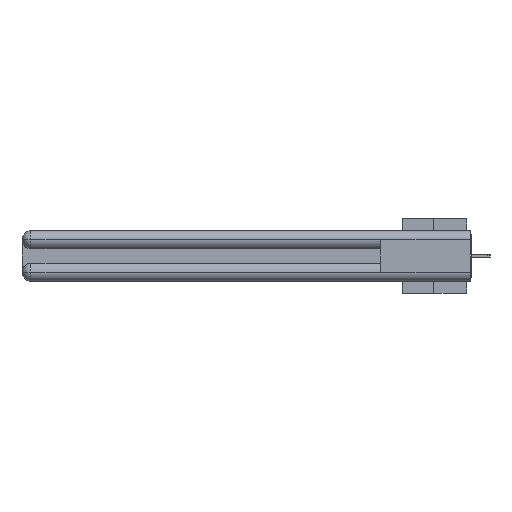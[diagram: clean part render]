
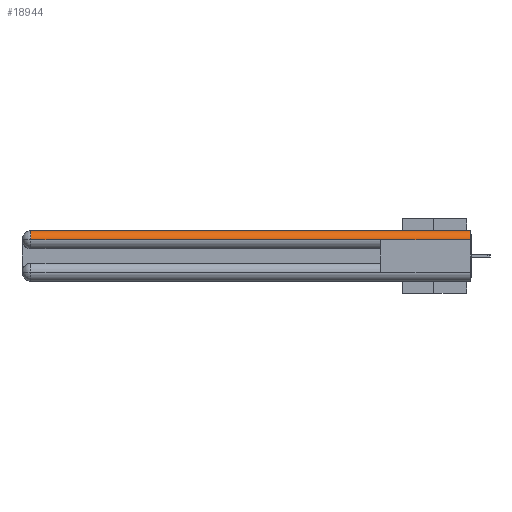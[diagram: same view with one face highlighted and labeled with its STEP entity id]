
A CAD part, left-side view. The second image highlights one B-rep face of the part: STEP entity #18944.
In plain terms, the highlighted cylindrical face has radius 1.562 mm (diameter 3.124 mm), a partial arc.
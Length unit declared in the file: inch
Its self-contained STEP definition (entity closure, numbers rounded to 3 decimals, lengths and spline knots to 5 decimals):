
#918 = VECTOR ( 'NONE', #4419, 39.37008 ) ;
#998 = CARTESIAN_POINT ( 'NONE',  ( 0., 2.94, -0.0615 ) ) ;
#1671 = VERTEX_POINT ( 'NONE', #998 ) ;
#1711 = CARTESIAN_POINT ( 'NONE',  ( 0., 3., -0.0615 ) ) ;
#1895 = LINE ( 'NONE', #37613, #918 ) ;
#2696 = VECTOR ( 'NONE', #34983, 39.37008 ) ;
#2831 = DIRECTION ( 'NONE',  ( 0., 1., 0. ) ) ;
#3626 = EDGE_LOOP ( 'NONE', ( #18050, #6326, #10313, #36601, #21862 ) ) ;
#4405 = DIRECTION ( 'NONE',  ( 0., 0., 1. ) ) ;
#4419 = DIRECTION ( 'NONE',  ( 0., -1., 0. ) ) ;
#4602 = CIRCLE ( 'NONE', #13078, 0.0615 ) ;
#5940 = CARTESIAN_POINT ( 'NONE',  ( 0.0615, 0., 0. ) ) ;
#6230 = CARTESIAN_POINT ( 'NONE',  ( 0.0615, 0., -0.0615 ) ) ;
#6326 = ORIENTED_EDGE ( 'NONE', *, *, #23701, .T. ) ;
#7381 = CARTESIAN_POINT ( 'NONE',  ( 0.0615, 0., -0.0615 ) ) ;
#8300 = VERTEX_POINT ( 'NONE', #18776 ) ;
#9349 = DIRECTION ( 'NONE',  ( 1., 0., 0. ) ) ;
#10313 = ORIENTED_EDGE ( 'NONE', *, *, #11606, .T. ) ;
#10641 = DIRECTION ( 'NONE',  ( 0., 1., 0. ) ) ;
#11606 = EDGE_CURVE ( 'NONE', #1671, #30646, #26923, .T. ) ;
#13078 = AXIS2_PLACEMENT_3D ( 'NONE', #14600, #35632, #17632 ) ;
#14280 = EDGE_CURVE ( 'NONE', #38505, #29261, #17786, .T. ) ;
#14600 = CARTESIAN_POINT ( 'NONE',  ( 0.0615, 2.94, -0.0615 ) ) ;
#14851 = AXIS2_PLACEMENT_3D ( 'NONE', #6230, #27400, #9349 ) ;
#17632 = DIRECTION ( 'NONE',  ( 0., 0., 1. ) ) ;
#17786 = CIRCLE ( 'NONE', #14851, 0.0615 ) ;
#18050 = ORIENTED_EDGE ( 'NONE', *, *, #21656, .F. ) ;
#18776 = CARTESIAN_POINT ( 'NONE',  ( 0.0615, 2.94, 0. ) ) ;
#18944 = ADVANCED_FACE ( 'NONE', ( #22563 ), #29571, .T. ) ;
#21105 = CARTESIAN_POINT ( 'NONE',  ( 0., 3., -0.0615 ) ) ;
#21656 = EDGE_CURVE ( 'NONE', #8300, #38505, #1895, .T. ) ;
#21862 = ORIENTED_EDGE ( 'NONE', *, *, #14280, .F. ) ;
#22563 = FACE_OUTER_BOUND ( 'NONE', #3626, .T. ) ;
#23701 = EDGE_CURVE ( 'NONE', #8300, #1671, #4602, .T. ) ;
#24674 = VECTOR ( 'NONE', #2831, 39.37008 ) ;
#26923 = LINE ( 'NONE', #1711, #2696 ) ;
#27400 = DIRECTION ( 'NONE',  ( 0., -1., 0. ) ) ;
#29261 = VERTEX_POINT ( 'NONE', #34579 ) ;
#29571 = CYLINDRICAL_SURFACE ( 'NONE', #37141, 0.0615 ) ;
#30646 = VERTEX_POINT ( 'NONE', #35661 ) ;
#31724 = LINE ( 'NONE', #21105, #24674 ) ;
#34579 = CARTESIAN_POINT ( 'NONE',  ( 0., 0., -0.0615 ) ) ;
#34983 = DIRECTION ( 'NONE',  ( 0., -1., 0. ) ) ;
#35632 = DIRECTION ( 'NONE',  ( 0., -1., 0. ) ) ;
#35661 = CARTESIAN_POINT ( 'NONE',  ( 0., 0.6, -0.0615 ) ) ;
#36601 = ORIENTED_EDGE ( 'NONE', *, *, #38471, .F. ) ;
#37141 = AXIS2_PLACEMENT_3D ( 'NONE', #7381, #10641, #4405 ) ;
#37613 = CARTESIAN_POINT ( 'NONE',  ( 0.0615, 0., 0. ) ) ;
#38471 = EDGE_CURVE ( 'NONE', #29261, #30646, #31724, .T. ) ;
#38505 = VERTEX_POINT ( 'NONE', #5940 ) ;
